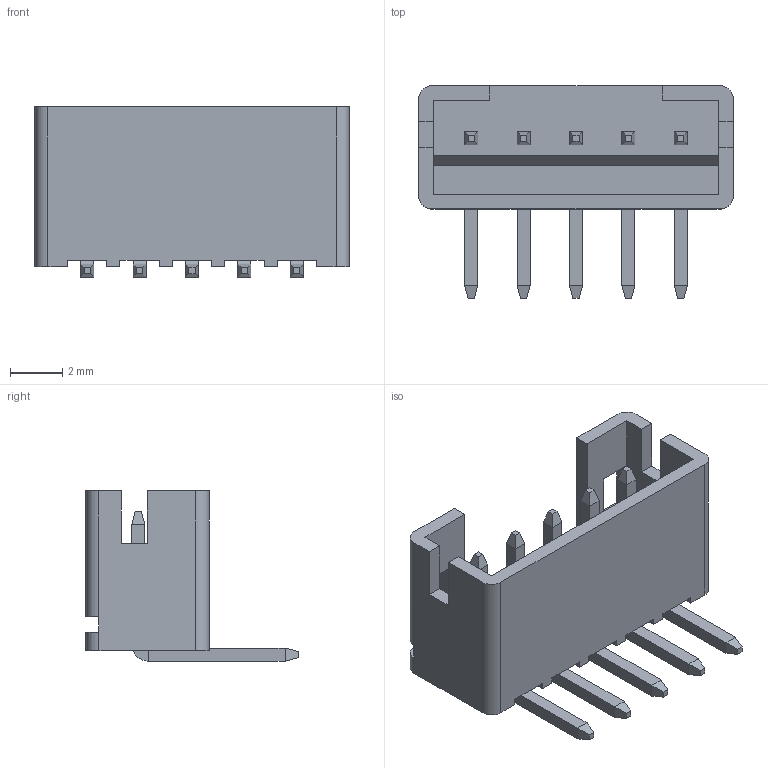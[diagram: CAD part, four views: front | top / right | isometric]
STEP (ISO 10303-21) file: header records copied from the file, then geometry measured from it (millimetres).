
FILE_DESCRIPTION (( 'STEP AP203' ), '1' );
FILE_NAME ('140-505-415-100.STEP', '2020-09-25T10:59:31', ( '' ), ( '' ), 'SwSTEP 2.0', 'SolidWorks 2020', '' );
FILE_SCHEMA (( 'CONFIG_CONTROL_DESIGN' ));
Length unit declared in the file: millimetre
Products named in the file (3): RA LI Housing_505; 140-505-415-100; RA LI Contact_Str
Assembly tree (6 placements, depth 2):
  140-505-415-100
    RA LI Housing_505
    RA LI Contact_Str  x5
Bounding box: 12 x 8.1 x 6.5 mm (x, y, z)
Volume: 141.4 mm3; surface area: 534.7 mm2
Topology: 6 solids, 6 shells, 190 faces, 456 edges, 276 vertices
Faces by surface type: plane 174, cylinder 16
Entity records: 3621 total; most frequent: CARTESIAN_POINT 571, ORIENTED_EDGE 560, DIRECTION 518, EDGE_CURVE 280, VECTOR 264, LINE 264, VERTEX_POINT 180, AXIS2_PLACEMENT_3D 127
